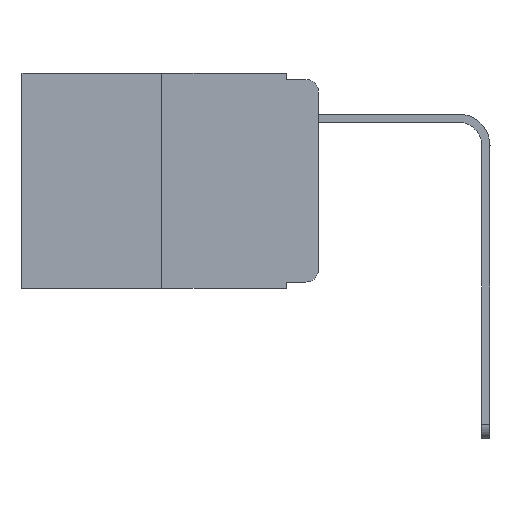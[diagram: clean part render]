
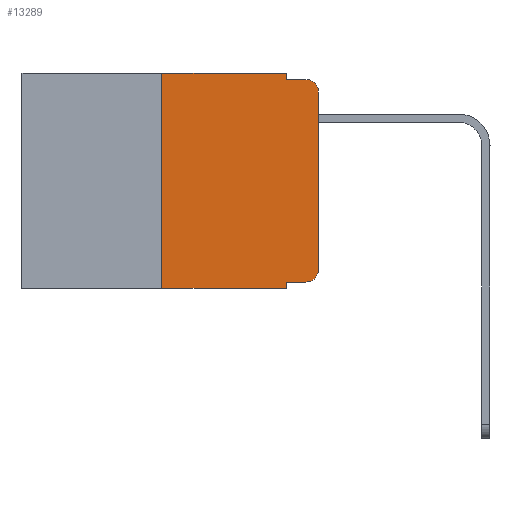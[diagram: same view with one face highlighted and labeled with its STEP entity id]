
A CAD part, left-side view. The second image highlights one B-rep face of the part: STEP entity #13289.
In plain terms, the highlighted planar face has unit normal (-1, 0, 0).
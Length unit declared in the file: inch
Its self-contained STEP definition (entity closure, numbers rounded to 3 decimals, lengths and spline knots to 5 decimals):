
#38 = EDGE_CURVE ( 'NONE', #15165, #2658, #11940, .T. ) ;
#379 = CARTESIAN_POINT ( 'NONE',  ( 0., 0., 0. ) ) ;
#469 = EDGE_CURVE ( 'NONE', #20371, #12216, #18495, .T. ) ;
#774 = VERTEX_POINT ( 'NONE', #3414 ) ;
#995 = CARTESIAN_POINT ( 'NONE',  ( 0., 0.02, -0.333 ) ) ;
#1315 = DIRECTION ( 'NONE',  ( 0., 0., -1. ) ) ;
#1363 = EDGE_CURVE ( 'NONE', #774, #3047, #12196, .T. ) ;
#1492 = CARTESIAN_POINT ( 'NONE',  ( 0., 0.051, -0.01 ) ) ;
#2604 = CARTESIAN_POINT ( 'NONE',  ( 0., 0.051, 0. ) ) ;
#2658 = VERTEX_POINT ( 'NONE', #6483 ) ;
#2675 = CARTESIAN_POINT ( 'NONE',  ( 0., 0.051, -0.343 ) ) ;
#2844 = EDGE_CURVE ( 'NONE', #774, #8819, #17642, .T. ) ;
#2936 = DIRECTION ( 'NONE',  ( 0., 0., -1. ) ) ;
#3003 = PLANE ( 'NONE',  #17872 ) ;
#3047 = VERTEX_POINT ( 'NONE', #8475 ) ;
#3066 = DIRECTION ( 'NONE',  ( 0., -1., 0. ) ) ;
#3238 = ORIENTED_EDGE ( 'NONE', *, *, #9551, .F. ) ;
#3326 = EDGE_LOOP ( 'NONE', ( #9910, #21448, #10149, #3238, #13909, #16756, #18011, #16590, #9357, #8530 ) ) ;
#3414 = CARTESIAN_POINT ( 'NONE',  ( 0., 0.25, -0.343 ) ) ;
#3953 = CARTESIAN_POINT ( 'NONE',  ( 0., 0.051, -0.333 ) ) ;
#3996 = VECTOR ( 'NONE', #13623, 39.37008 ) ;
#3999 = CIRCLE ( 'NONE', #19592, 0.02 ) ;
#4659 = DIRECTION ( 'NONE',  ( 0., 0., -1. ) ) ;
#4795 = VECTOR ( 'NONE', #13716, 39.37008 ) ;
#4821 = LINE ( 'NONE', #13830, #20396 ) ;
#5232 = FACE_OUTER_BOUND ( 'NONE', #3326, .T. ) ;
#5385 = LINE ( 'NONE', #2604, #9469 ) ;
#5980 = VERTEX_POINT ( 'NONE', #20966 ) ;
#6384 = DIRECTION ( 'NONE',  ( 0., -1., 0. ) ) ;
#6483 = CARTESIAN_POINT ( 'NONE',  ( 0., 0., -0.313 ) ) ;
#6882 = EDGE_CURVE ( 'NONE', #20104, #8819, #5385, .T. ) ;
#7661 = DIRECTION ( 'NONE',  ( -1., 0., 0. ) ) ;
#7997 = EDGE_CURVE ( 'NONE', #20104, #15165, #14396, .T. ) ;
#8061 = VECTOR ( 'NONE', #18704, 39.37008 ) ;
#8475 = CARTESIAN_POINT ( 'NONE',  ( 0., 0.25, 0. ) ) ;
#8530 = ORIENTED_EDGE ( 'NONE', *, *, #38, .T. ) ;
#8819 = VERTEX_POINT ( 'NONE', #2675 ) ;
#9357 = ORIENTED_EDGE ( 'NONE', *, *, #7997, .T. ) ;
#9469 = VECTOR ( 'NONE', #13219, 39.37008 ) ;
#9551 = EDGE_CURVE ( 'NONE', #12865, #20371, #17458, .T. ) ;
#9775 = CARTESIAN_POINT ( 'NONE',  ( 0., 0.02, -0.03 ) ) ;
#9910 = ORIENTED_EDGE ( 'NONE', *, *, #19421, .T. ) ;
#10026 = CARTESIAN_POINT ( 'NONE',  ( 0., 0.051, -0.333 ) ) ;
#10149 = ORIENTED_EDGE ( 'NONE', *, *, #469, .F. ) ;
#11794 = CARTESIAN_POINT ( 'NONE',  ( 0., 0.25, 0. ) ) ;
#11940 = CIRCLE ( 'NONE', #21174, 0.02 ) ;
#12196 = LINE ( 'NONE', #11794, #4795 ) ;
#12216 = VERTEX_POINT ( 'NONE', #14817 ) ;
#12865 = VERTEX_POINT ( 'NONE', #20513 ) ;
#13219 = DIRECTION ( 'NONE',  ( 0., 0., -1. ) ) ;
#13289 = ADVANCED_FACE ( 'NONE', ( #5232 ), #3003, .F. ) ;
#13320 = CARTESIAN_POINT ( 'NONE',  ( 0., 0.473, 0. ) ) ;
#13623 = DIRECTION ( 'NONE',  ( 0., -1., 0. ) ) ;
#13716 = DIRECTION ( 'NONE',  ( 0., 0., 1. ) ) ;
#13816 = VECTOR ( 'NONE', #3066, 39.37008 ) ;
#13830 = CARTESIAN_POINT ( 'NONE',  ( 0., 0.473, 0. ) ) ;
#13909 = ORIENTED_EDGE ( 'NONE', *, *, #21593, .F. ) ;
#14396 = LINE ( 'NONE', #10026, #18496 ) ;
#14446 = VECTOR ( 'NONE', #16915, 39.37008 ) ;
#14817 = CARTESIAN_POINT ( 'NONE',  ( 0., 0.02, -0.01 ) ) ;
#14907 = LINE ( 'NONE', #379, #8061 ) ;
#15165 = VERTEX_POINT ( 'NONE', #995 ) ;
#15479 = CARTESIAN_POINT ( 'NONE',  ( 0., 0.051, 0. ) ) ;
#15726 = DIRECTION ( 'NONE',  ( 0., -1., 0. ) ) ;
#16590 = ORIENTED_EDGE ( 'NONE', *, *, #6882, .F. ) ;
#16756 = ORIENTED_EDGE ( 'NONE', *, *, #1363, .F. ) ;
#16915 = DIRECTION ( 'NONE',  ( 0., 0., -1. ) ) ;
#17458 = LINE ( 'NONE', #15479, #14446 ) ;
#17642 = LINE ( 'NONE', #22147, #13816 ) ;
#17872 = AXIS2_PLACEMENT_3D ( 'NONE', #13320, #18514, #2936 ) ;
#18011 = ORIENTED_EDGE ( 'NONE', *, *, #2844, .T. ) ;
#18131 = CARTESIAN_POINT ( 'NONE',  ( 0., 0.02, -0.313 ) ) ;
#18494 = DIRECTION ( 'NONE',  ( -1., 0., 0. ) ) ;
#18495 = LINE ( 'NONE', #20478, #3996 ) ;
#18496 = VECTOR ( 'NONE', #6384, 39.37008 ) ;
#18514 = DIRECTION ( 'NONE',  ( 1., 0., 0. ) ) ;
#18704 = DIRECTION ( 'NONE',  ( 0., 0., 1. ) ) ;
#18863 = EDGE_CURVE ( 'NONE', #5980, #12216, #3999, .T. ) ;
#19421 = EDGE_CURVE ( 'NONE', #2658, #5980, #14907, .T. ) ;
#19592 = AXIS2_PLACEMENT_3D ( 'NONE', #9775, #18494, #4659 ) ;
#20104 = VERTEX_POINT ( 'NONE', #3953 ) ;
#20371 = VERTEX_POINT ( 'NONE', #1492 ) ;
#20396 = VECTOR ( 'NONE', #15726, 39.37008 ) ;
#20478 = CARTESIAN_POINT ( 'NONE',  ( 0., 0.051, -0.01 ) ) ;
#20513 = CARTESIAN_POINT ( 'NONE',  ( 0., 0.051, 0. ) ) ;
#20966 = CARTESIAN_POINT ( 'NONE',  ( 0., 0., -0.03 ) ) ;
#21174 = AXIS2_PLACEMENT_3D ( 'NONE', #18131, #7661, #1315 ) ;
#21448 = ORIENTED_EDGE ( 'NONE', *, *, #18863, .T. ) ;
#21593 = EDGE_CURVE ( 'NONE', #3047, #12865, #4821, .T. ) ;
#22147 = CARTESIAN_POINT ( 'NONE',  ( 0., 0.473, -0.343 ) ) ;
